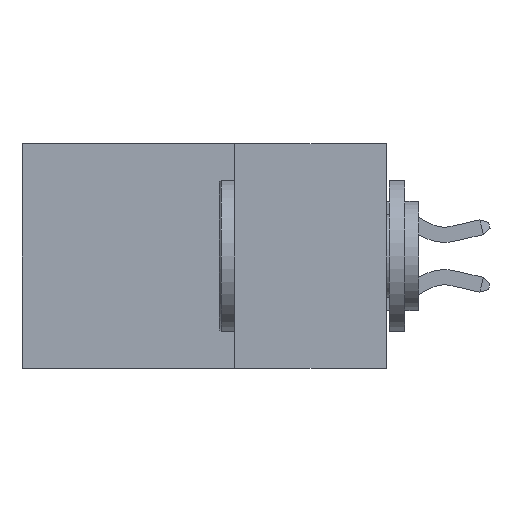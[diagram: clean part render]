
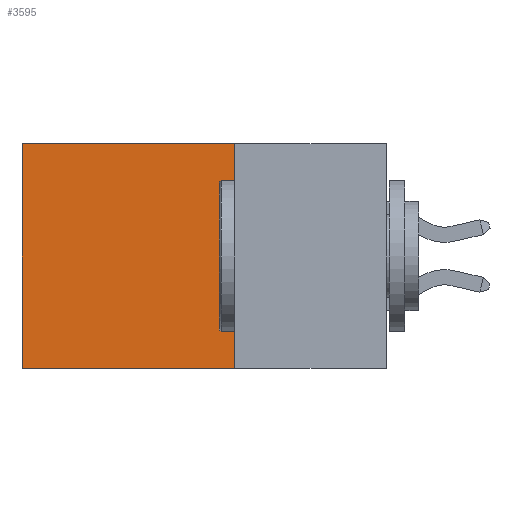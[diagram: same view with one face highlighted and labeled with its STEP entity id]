
A CAD part, left-side view. The second image highlights one B-rep face of the part: STEP entity #3595.
In plain terms, the highlighted planar face has unit normal (-1, 0, 0).
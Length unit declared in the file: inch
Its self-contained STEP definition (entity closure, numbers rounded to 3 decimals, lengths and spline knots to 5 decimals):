
#111 = VECTOR ( 'NONE', #1199, 39.37008 ) ;
#814 = ORIENTED_EDGE ( 'NONE', *, *, #1010, .F. ) ;
#1010 = EDGE_CURVE ( 'NONE', #2606, #2564, #1836, .T. ) ;
#1023 = DIRECTION ( 'NONE',  ( 0., 0., -1. ) ) ;
#1139 = CARTESIAN_POINT ( 'NONE',  ( 0.2615, 0.6, -0.37 ) ) ;
#1199 = DIRECTION ( 'NONE',  ( 0., 0., -1. ) ) ;
#1218 = CARTESIAN_POINT ( 'NONE',  ( 0.2615, 0.25, -0.37 ) ) ;
#1343 = LINE ( 'NONE', #6950, #111 ) ;
#1527 = DIRECTION ( 'NONE',  ( 0., 1., 0. ) ) ;
#1741 = EDGE_CURVE ( 'NONE', #2633, #2564, #1343, .T. ) ;
#1836 = LINE ( 'NONE', #8794, #13033 ) ;
#1967 = DIRECTION ( 'NONE',  ( 0., 1., 0. ) ) ;
#2564 = VERTEX_POINT ( 'NONE', #1139 ) ;
#2606 = VERTEX_POINT ( 'NONE', #1218 ) ;
#2633 = VERTEX_POINT ( 'NONE', #10748 ) ;
#2928 = DIRECTION ( 'NONE',  ( 1., 0., 0. ) ) ;
#2944 = LINE ( 'NONE', #8694, #4241 ) ;
#3595 = ADVANCED_FACE ( 'NONE', ( #4000 ), #8452, .F. ) ;
#4000 = FACE_OUTER_BOUND ( 'NONE', #7414, .T. ) ;
#4241 = VECTOR ( 'NONE', #1967, 39.37008 ) ;
#4445 = VECTOR ( 'NONE', #1023, 39.37008 ) ;
#4472 = ORIENTED_EDGE ( 'NONE', *, *, #1741, .T. ) ;
#6785 = EDGE_CURVE ( 'NONE', #12221, #2606, #8415, .T. ) ;
#6857 = CARTESIAN_POINT ( 'NONE',  ( 0.2615, 0.25, -0.37 ) ) ;
#6950 = CARTESIAN_POINT ( 'NONE',  ( 0.2615, 0.6, -0.37 ) ) ;
#7414 = EDGE_LOOP ( 'NONE', ( #4472, #814, #13078, #10340 ) ) ;
#7456 = DIRECTION ( 'NONE',  ( 0., 0., -1. ) ) ;
#8415 = LINE ( 'NONE', #6857, #4445 ) ;
#8452 = PLANE ( 'NONE',  #13565 ) ;
#8694 = CARTESIAN_POINT ( 'NONE',  ( 0.2615, 0.25, 0. ) ) ;
#8700 = CARTESIAN_POINT ( 'NONE',  ( 0.2615, 0.25, 0. ) ) ;
#8794 = CARTESIAN_POINT ( 'NONE',  ( 0.2615, 0.25, -0.37 ) ) ;
#9099 = EDGE_CURVE ( 'NONE', #12221, #2633, #2944, .T. ) ;
#10340 = ORIENTED_EDGE ( 'NONE', *, *, #9099, .T. ) ;
#10748 = CARTESIAN_POINT ( 'NONE',  ( 0.2615, 0.6, 0. ) ) ;
#12018 = CARTESIAN_POINT ( 'NONE',  ( 0.2615, 0.25, -0.37 ) ) ;
#12221 = VERTEX_POINT ( 'NONE', #8700 ) ;
#13033 = VECTOR ( 'NONE', #1527, 39.37008 ) ;
#13078 = ORIENTED_EDGE ( 'NONE', *, *, #6785, .F. ) ;
#13565 = AXIS2_PLACEMENT_3D ( 'NONE', #12018, #2928, #7456 ) ;
